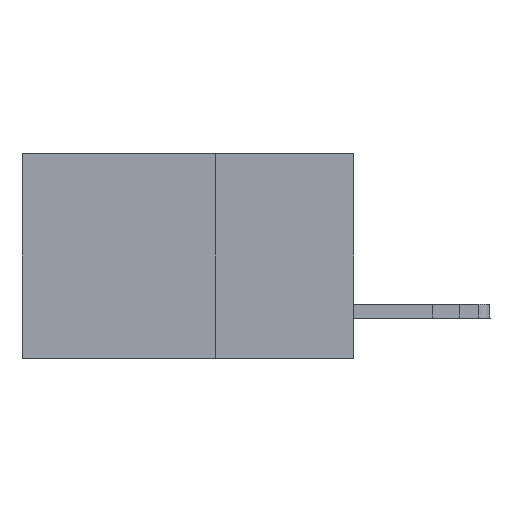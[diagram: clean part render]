
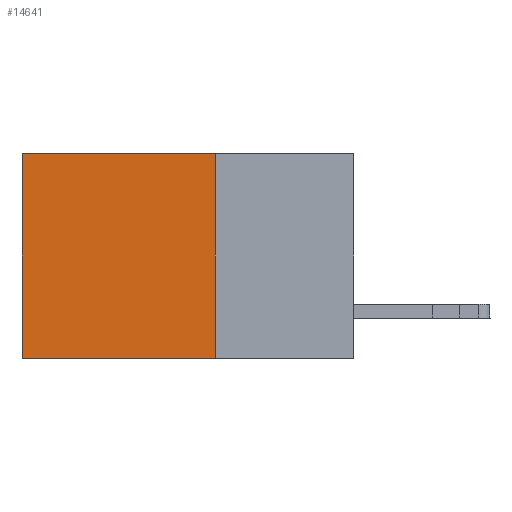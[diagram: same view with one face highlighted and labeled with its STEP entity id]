
A CAD part, left-side view. The second image highlights one B-rep face of the part: STEP entity #14641.
In plain terms, the highlighted planar face has unit normal (-1, 0, 0).
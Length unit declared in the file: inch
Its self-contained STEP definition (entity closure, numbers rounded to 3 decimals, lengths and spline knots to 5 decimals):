
#143 = ORIENTED_EDGE ( 'NONE', *, *, #12355, .T. ) ;
#152 = LINE ( 'NONE', #14182, #12337 ) ;
#441 = DIRECTION ( 'NONE',  ( 0., 0., -1. ) ) ;
#532 = CARTESIAN_POINT ( 'NONE',  ( 0.2875, 0.6, 0. ) ) ;
#1218 = ORIENTED_EDGE ( 'NONE', *, *, #2178, .F. ) ;
#1723 = VECTOR ( 'NONE', #11660, 39.37008 ) ;
#2178 = EDGE_CURVE ( 'NONE', #17627, #14460, #14957, .T. ) ;
#3282 = LINE ( 'NONE', #3495, #10220 ) ;
#3495 = CARTESIAN_POINT ( 'NONE',  ( 0.2875, 0.25, 0. ) ) ;
#4211 = CARTESIAN_POINT ( 'NONE',  ( 0.2875, 0.25, 0. ) ) ;
#4921 = CARTESIAN_POINT ( 'NONE',  ( 0.2875, 0.25, -0.37 ) ) ;
#5157 = CARTESIAN_POINT ( 'NONE',  ( 0.2875, 0.25, 0. ) ) ;
#5294 = FACE_OUTER_BOUND ( 'NONE', #8152, .T. ) ;
#6082 = VECTOR ( 'NONE', #14257, 39.37008 ) ;
#6231 = CARTESIAN_POINT ( 'NONE',  ( 0.2875, 0.6, -0.37 ) ) ;
#6397 = AXIS2_PLACEMENT_3D ( 'NONE', #9708, #8510, #15824 ) ;
#8152 = EDGE_LOOP ( 'NONE', ( #143, #14322, #1218, #14093 ) ) ;
#8510 = DIRECTION ( 'NONE',  ( 1., 0., 0. ) ) ;
#9525 = DIRECTION ( 'NONE',  ( 0., 1., 0. ) ) ;
#9708 = CARTESIAN_POINT ( 'NONE',  ( 0.2875, 0.25, 0. ) ) ;
#10220 = VECTOR ( 'NONE', #9525, 39.37008 ) ;
#11660 = DIRECTION ( 'NONE',  ( 0., 0., -1. ) ) ;
#12337 = VECTOR ( 'NONE', #441, 39.37008 ) ;
#12352 = LINE ( 'NONE', #4921, #6082 ) ;
#12355 = EDGE_CURVE ( 'NONE', #15297, #17139, #152, .T. ) ;
#13119 = PLANE ( 'NONE',  #6397 ) ;
#14093 = ORIENTED_EDGE ( 'NONE', *, *, #14472, .T. ) ;
#14104 = EDGE_CURVE ( 'NONE', #14460, #17139, #12352, .T. ) ;
#14182 = CARTESIAN_POINT ( 'NONE',  ( 0.2875, 0.6, 0. ) ) ;
#14257 = DIRECTION ( 'NONE',  ( 0., 1., 0. ) ) ;
#14322 = ORIENTED_EDGE ( 'NONE', *, *, #14104, .F. ) ;
#14460 = VERTEX_POINT ( 'NONE', #17024 ) ;
#14472 = EDGE_CURVE ( 'NONE', #17627, #15297, #3282, .T. ) ;
#14641 = ADVANCED_FACE ( 'NONE', ( #5294 ), #13119, .F. ) ;
#14957 = LINE ( 'NONE', #4211, #1723 ) ;
#15297 = VERTEX_POINT ( 'NONE', #532 ) ;
#15824 = DIRECTION ( 'NONE',  ( 0., 0., -1. ) ) ;
#17024 = CARTESIAN_POINT ( 'NONE',  ( 0.2875, 0.25, -0.37 ) ) ;
#17139 = VERTEX_POINT ( 'NONE', #6231 ) ;
#17627 = VERTEX_POINT ( 'NONE', #5157 ) ;
